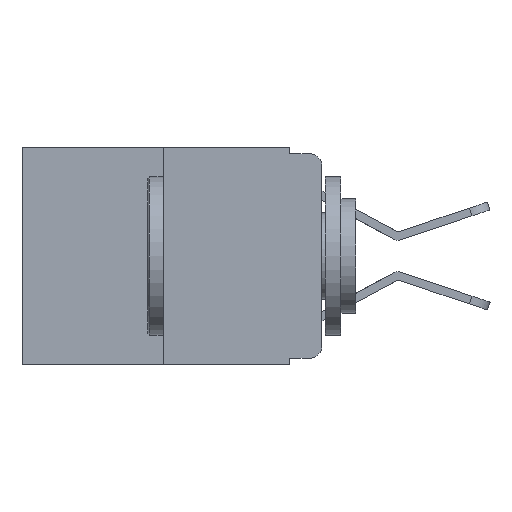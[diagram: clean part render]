
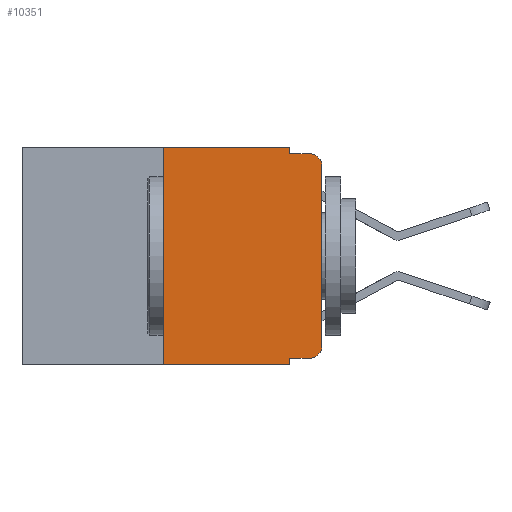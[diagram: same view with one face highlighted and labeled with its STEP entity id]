
A CAD part, left-side view. The second image highlights one B-rep face of the part: STEP entity #10351.
In plain terms, the highlighted planar face has unit normal (-1, 0, 0).
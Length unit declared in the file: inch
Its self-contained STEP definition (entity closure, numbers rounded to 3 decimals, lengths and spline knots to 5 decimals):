
#169 = VERTEX_POINT ( 'NONE', #6583 ) ;
#261 = EDGE_CURVE ( 'NONE', #13080, #12245, #4455, .T. ) ;
#491 = ORIENTED_EDGE ( 'NONE', *, *, #14143, .F. ) ;
#622 = DIRECTION ( 'NONE',  ( -1., 0., 0. ) ) ;
#762 = LINE ( 'NONE', #15584, #2315 ) ;
#1081 = CARTESIAN_POINT ( 'NONE',  ( 0., 0., 0. ) ) ;
#1274 = VERTEX_POINT ( 'NONE', #7599 ) ;
#1463 = ORIENTED_EDGE ( 'NONE', *, *, #13145, .T. ) ;
#1826 = CARTESIAN_POINT ( 'NONE',  ( 0., 0.25, -0.343 ) ) ;
#2007 = DIRECTION ( 'NONE',  ( 0., 0., -1. ) ) ;
#2256 = VERTEX_POINT ( 'NONE', #3831 ) ;
#2315 = VECTOR ( 'NONE', #10581, 39.37008 ) ;
#2456 = CARTESIAN_POINT ( 'NONE',  ( 0., 0.02, -0.333 ) ) ;
#2594 = AXIS2_PLACEMENT_3D ( 'NONE', #3325, #14476, #10866 ) ;
#2741 = VECTOR ( 'NONE', #7825, 39.37008 ) ;
#3007 = CARTESIAN_POINT ( 'NONE',  ( 0., 0.02, -0.313 ) ) ;
#3078 = EDGE_CURVE ( 'NONE', #6176, #12245, #762, .T. ) ;
#3325 = CARTESIAN_POINT ( 'NONE',  ( 0., 0.473, 0. ) ) ;
#3831 = CARTESIAN_POINT ( 'NONE',  ( 0., 0.25, 0. ) ) ;
#4004 = EDGE_CURVE ( 'NONE', #2256, #1274, #15607, .T. ) ;
#4101 = VECTOR ( 'NONE', #9571, 39.37008 ) ;
#4455 = LINE ( 'NONE', #7385, #11426 ) ;
#4551 = CARTESIAN_POINT ( 'NONE',  ( 0., 0.051, -0.333 ) ) ;
#4760 = FACE_OUTER_BOUND ( 'NONE', #9956, .T. ) ;
#4843 = CARTESIAN_POINT ( 'NONE',  ( 0., 0.051, -0.333 ) ) ;
#4858 = LINE ( 'NONE', #5316, #2741 ) ;
#4917 = VERTEX_POINT ( 'NONE', #9194 ) ;
#5316 = CARTESIAN_POINT ( 'NONE',  ( 0., 0.051, 0. ) ) ;
#5325 = CIRCLE ( 'NONE', #14020, 0.02 ) ;
#5341 = CARTESIAN_POINT ( 'NONE',  ( 0., 0.473, 0. ) ) ;
#5392 = DIRECTION ( 'NONE',  ( 0., -1., 0. ) ) ;
#5800 = DIRECTION ( 'NONE',  ( -1., 0., 0. ) ) ;
#6176 = VERTEX_POINT ( 'NONE', #1826 ) ;
#6307 = EDGE_CURVE ( 'NONE', #6176, #2256, #6504, .T. ) ;
#6367 = ORIENTED_EDGE ( 'NONE', *, *, #6802, .T. ) ;
#6434 = LINE ( 'NONE', #4551, #7201 ) ;
#6504 = LINE ( 'NONE', #11659, #9578 ) ;
#6583 = CARTESIAN_POINT ( 'NONE',  ( 0., 0., -0.313 ) ) ;
#6793 = VECTOR ( 'NONE', #13057, 39.37008 ) ;
#6802 = EDGE_CURVE ( 'NONE', #7209, #169, #5325, .T. ) ;
#7201 = VECTOR ( 'NONE', #8050, 39.37008 ) ;
#7209 = VERTEX_POINT ( 'NONE', #2456 ) ;
#7385 = CARTESIAN_POINT ( 'NONE',  ( 0., 0.051, 0. ) ) ;
#7412 = ORIENTED_EDGE ( 'NONE', *, *, #6307, .F. ) ;
#7599 = CARTESIAN_POINT ( 'NONE',  ( 0., 0.051, 0. ) ) ;
#7649 = EDGE_CURVE ( 'NONE', #4917, #13877, #14753, .T. ) ;
#7825 = DIRECTION ( 'NONE',  ( 0., 0., -1. ) ) ;
#7857 = DIRECTION ( 'NONE',  ( 0., 0., -1. ) ) ;
#8050 = DIRECTION ( 'NONE',  ( 0., -1., 0. ) ) ;
#8079 = CARTESIAN_POINT ( 'NONE',  ( 0., 0.051, -0.01 ) ) ;
#8579 = CARTESIAN_POINT ( 'NONE',  ( 0., 0.051, -0.01 ) ) ;
#8608 = ORIENTED_EDGE ( 'NONE', *, *, #3078, .T. ) ;
#9194 = CARTESIAN_POINT ( 'NONE',  ( 0., 0., -0.03 ) ) ;
#9571 = DIRECTION ( 'NONE',  ( 0., 0., 1. ) ) ;
#9578 = VECTOR ( 'NONE', #15362, 39.37008 ) ;
#9956 = EDGE_LOOP ( 'NONE', ( #12304, #14591, #491, #14204, #11097, #7412, #8608, #15009, #1463, #6367 ) ) ;
#10214 = CARTESIAN_POINT ( 'NONE',  ( 0., 0.051, -0.343 ) ) ;
#10351 = ADVANCED_FACE ( 'NONE', ( #4760 ), #13401, .F. ) ;
#10581 = DIRECTION ( 'NONE',  ( 0., -1., 0. ) ) ;
#10851 = CARTESIAN_POINT ( 'NONE',  ( 0., 0.02, -0.03 ) ) ;
#10866 = DIRECTION ( 'NONE',  ( 0., 0., -1. ) ) ;
#11000 = VECTOR ( 'NONE', #5392, 39.37008 ) ;
#11097 = ORIENTED_EDGE ( 'NONE', *, *, #4004, .F. ) ;
#11426 = VECTOR ( 'NONE', #13366, 39.37008 ) ;
#11451 = LINE ( 'NONE', #1081, #4101 ) ;
#11659 = CARTESIAN_POINT ( 'NONE',  ( 0., 0.25, 0. ) ) ;
#11744 = AXIS2_PLACEMENT_3D ( 'NONE', #10851, #5800, #2007 ) ;
#12245 = VERTEX_POINT ( 'NONE', #10214 ) ;
#12304 = ORIENTED_EDGE ( 'NONE', *, *, #13796, .T. ) ;
#12423 = CARTESIAN_POINT ( 'NONE',  ( 0., 0.02, -0.01 ) ) ;
#12663 = VERTEX_POINT ( 'NONE', #8579 ) ;
#13057 = DIRECTION ( 'NONE',  ( 0., -1., 0. ) ) ;
#13080 = VERTEX_POINT ( 'NONE', #4843 ) ;
#13145 = EDGE_CURVE ( 'NONE', #13080, #7209, #6434, .T. ) ;
#13366 = DIRECTION ( 'NONE',  ( 0., 0., -1. ) ) ;
#13401 = PLANE ( 'NONE',  #2594 ) ;
#13796 = EDGE_CURVE ( 'NONE', #169, #4917, #11451, .T. ) ;
#13877 = VERTEX_POINT ( 'NONE', #12423 ) ;
#14020 = AXIS2_PLACEMENT_3D ( 'NONE', #3007, #622, #7857 ) ;
#14084 = EDGE_CURVE ( 'NONE', #1274, #12663, #4858, .T. ) ;
#14143 = EDGE_CURVE ( 'NONE', #12663, #13877, #14881, .T. ) ;
#14204 = ORIENTED_EDGE ( 'NONE', *, *, #14084, .F. ) ;
#14476 = DIRECTION ( 'NONE',  ( 1., 0., 0. ) ) ;
#14591 = ORIENTED_EDGE ( 'NONE', *, *, #7649, .T. ) ;
#14753 = CIRCLE ( 'NONE', #11744, 0.02 ) ;
#14881 = LINE ( 'NONE', #8079, #6793 ) ;
#15009 = ORIENTED_EDGE ( 'NONE', *, *, #261, .F. ) ;
#15362 = DIRECTION ( 'NONE',  ( 0., 0., 1. ) ) ;
#15584 = CARTESIAN_POINT ( 'NONE',  ( 0., 0.473, -0.343 ) ) ;
#15607 = LINE ( 'NONE', #5341, #11000 ) ;
